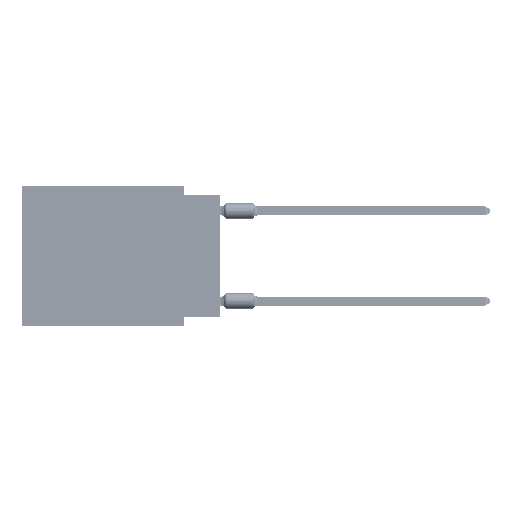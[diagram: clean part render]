
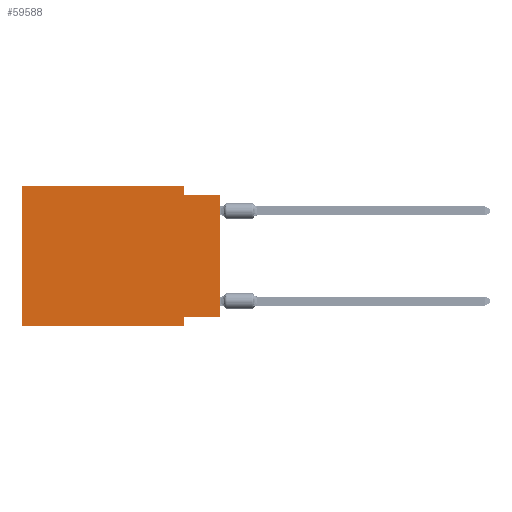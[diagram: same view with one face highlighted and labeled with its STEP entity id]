
A CAD part, left-side view. The second image highlights one B-rep face of the part: STEP entity #59588.
In plain terms, the highlighted planar face has unit normal (-1, 0, 0).
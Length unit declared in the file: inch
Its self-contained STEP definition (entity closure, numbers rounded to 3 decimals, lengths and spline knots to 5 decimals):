
#1121 = ORIENTED_EDGE ( 'NONE', *, *, #14769, .T. ) ;
#1270 = CARTESIAN_POINT ( 'NONE',  ( 0., 0.1, -0.39 ) ) ;
#2849 = ORIENTED_EDGE ( 'NONE', *, *, #57645, .F. ) ;
#4646 = CARTESIAN_POINT ( 'NONE',  ( 0., 0.1, -0.025 ) ) ;
#5534 = VERTEX_POINT ( 'NONE', #66538 ) ;
#6573 = CARTESIAN_POINT ( 'NONE',  ( 0., 0.55, -0.39 ) ) ;
#8178 = PLANE ( 'NONE',  #67068 ) ;
#9328 = FACE_OUTER_BOUND ( 'NONE', #13598, .T. ) ;
#9391 = CARTESIAN_POINT ( 'NONE',  ( 0., 0.1, 0. ) ) ;
#13244 = CARTESIAN_POINT ( 'NONE',  ( 0., 0.55, 0. ) ) ;
#13490 = CARTESIAN_POINT ( 'NONE',  ( 0., 0.55, 0. ) ) ;
#13598 = EDGE_LOOP ( 'NONE', ( #50491, #55234, #2849, #49372, #53875, #1121, #31886, #67320 ) ) ;
#14769 = EDGE_CURVE ( 'NONE', #17712, #26647, #18097, .T. ) ;
#15648 = EDGE_CURVE ( 'NONE', #5534, #26647, #18944, .T. ) ;
#16002 = LINE ( 'NONE', #34436, #33154 ) ;
#17712 = VERTEX_POINT ( 'NONE', #57263 ) ;
#18097 = LINE ( 'NONE', #6573, #65852 ) ;
#18944 = LINE ( 'NONE', #59336, #31343 ) ;
#21727 = LINE ( 'NONE', #46307, #28778 ) ;
#22720 = LINE ( 'NONE', #47298, #55239 ) ;
#25470 = DIRECTION ( 'NONE',  ( 1., 0., 0. ) ) ;
#25851 = CARTESIAN_POINT ( 'NONE',  ( 0., 0.55, 0. ) ) ;
#26647 = VERTEX_POINT ( 'NONE', #1270 ) ;
#28727 = VERTEX_POINT ( 'NONE', #4646 ) ;
#28778 = VECTOR ( 'NONE', #51326, 39.37008 ) ;
#30114 = VERTEX_POINT ( 'NONE', #9391 ) ;
#31343 = VECTOR ( 'NONE', #36232, 39.37008 ) ;
#31886 = ORIENTED_EDGE ( 'NONE', *, *, #15648, .F. ) ;
#31931 = LINE ( 'NONE', #13490, #74815 ) ;
#32191 = VERTEX_POINT ( 'NONE', #57604 ) ;
#32679 = EDGE_CURVE ( 'NONE', #48921, #30114, #16002, .T. ) ;
#33154 = VECTOR ( 'NONE', #57895, 39.37008 ) ;
#34436 = CARTESIAN_POINT ( 'NONE',  ( 0., 0.55, 0. ) ) ;
#34611 = CARTESIAN_POINT ( 'NONE',  ( 0., 0., -0.025 ) ) ;
#36232 = DIRECTION ( 'NONE',  ( 0., 0., -1. ) ) ;
#36929 = DIRECTION ( 'NONE',  ( 0., 0., 1. ) ) ;
#37206 = EDGE_CURVE ( 'NONE', #28727, #50881, #45782, .T. ) ;
#38445 = EDGE_CURVE ( 'NONE', #32191, #5534, #22720, .T. ) ;
#38608 = VECTOR ( 'NONE', #75951, 39.37008 ) ;
#41546 = DIRECTION ( 'NONE',  ( 0., -1., 0. ) ) ;
#42070 = CARTESIAN_POINT ( 'NONE',  ( 0., 0.1, 0. ) ) ;
#44687 = DIRECTION ( 'NONE',  ( 0., 0., -1. ) ) ;
#45782 = LINE ( 'NONE', #34611, #53241 ) ;
#46307 = CARTESIAN_POINT ( 'NONE',  ( 0., 0., 0. ) ) ;
#46526 = DIRECTION ( 'NONE',  ( 0., -1., 0. ) ) ;
#47298 = CARTESIAN_POINT ( 'NONE',  ( 0., 0., -0.365 ) ) ;
#47573 = EDGE_CURVE ( 'NONE', #32191, #50881, #21727, .T. ) ;
#48921 = VERTEX_POINT ( 'NONE', #13244 ) ;
#49372 = ORIENTED_EDGE ( 'NONE', *, *, #32679, .F. ) ;
#50491 = ORIENTED_EDGE ( 'NONE', *, *, #47573, .T. ) ;
#50881 = VERTEX_POINT ( 'NONE', #59250 ) ;
#51326 = DIRECTION ( 'NONE',  ( 0., 0., 1. ) ) ;
#52686 = DIRECTION ( 'NONE',  ( 0., 1., 0. ) ) ;
#53241 = VECTOR ( 'NONE', #46526, 39.37008 ) ;
#53875 = ORIENTED_EDGE ( 'NONE', *, *, #70117, .F. ) ;
#55234 = ORIENTED_EDGE ( 'NONE', *, *, #37206, .F. ) ;
#55239 = VECTOR ( 'NONE', #52686, 39.37008 ) ;
#57263 = CARTESIAN_POINT ( 'NONE',  ( 0., 0.55, -0.39 ) ) ;
#57604 = CARTESIAN_POINT ( 'NONE',  ( 0., 0., -0.365 ) ) ;
#57645 = EDGE_CURVE ( 'NONE', #30114, #28727, #58249, .T. ) ;
#57895 = DIRECTION ( 'NONE',  ( 0., -1., 0. ) ) ;
#58249 = LINE ( 'NONE', #42070, #38608 ) ;
#59250 = CARTESIAN_POINT ( 'NONE',  ( 0., 0., -0.025 ) ) ;
#59336 = CARTESIAN_POINT ( 'NONE',  ( 0., 0.1, -0.39 ) ) ;
#59588 = ADVANCED_FACE ( 'NONE', ( #9328 ), #8178, .F. ) ;
#65852 = VECTOR ( 'NONE', #41546, 39.37008 ) ;
#66538 = CARTESIAN_POINT ( 'NONE',  ( 0., 0.1, -0.365 ) ) ;
#67068 = AXIS2_PLACEMENT_3D ( 'NONE', #25851, #25470, #44687 ) ;
#67320 = ORIENTED_EDGE ( 'NONE', *, *, #38445, .F. ) ;
#70117 = EDGE_CURVE ( 'NONE', #17712, #48921, #31931, .T. ) ;
#74815 = VECTOR ( 'NONE', #36929, 39.37008 ) ;
#75951 = DIRECTION ( 'NONE',  ( 0., 0., -1. ) ) ;
